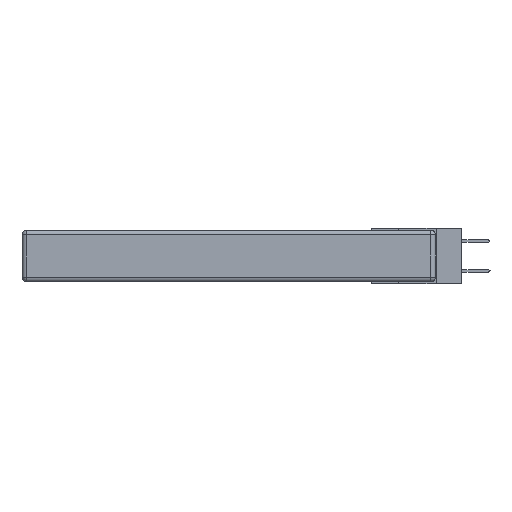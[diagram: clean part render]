
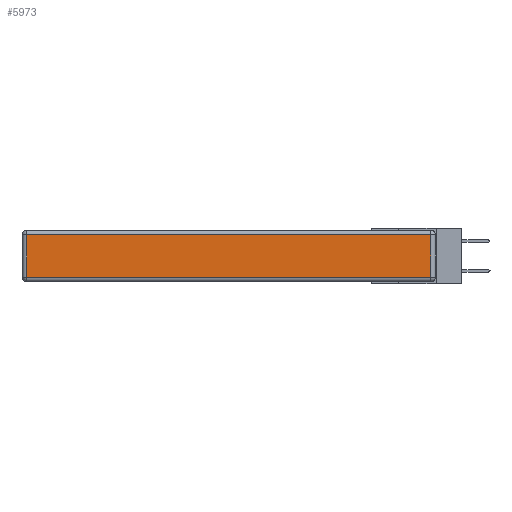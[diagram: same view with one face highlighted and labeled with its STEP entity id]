
A CAD part, left-side view. The second image highlights one B-rep face of the part: STEP entity #5973.
In plain terms, the highlighted planar face has unit normal (-1, 0, 0).
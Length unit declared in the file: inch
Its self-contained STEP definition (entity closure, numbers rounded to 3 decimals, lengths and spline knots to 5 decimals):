
#1012 = CARTESIAN_POINT ( 'NONE',  ( 0., 2.72, -0.313 ) ) ;
#1584 = VERTEX_POINT ( 'NONE', #6991 ) ;
#1770 = EDGE_CURVE ( 'NONE', #4336, #4052, #16063, .T. ) ;
#3275 = LINE ( 'NONE', #14024, #15629 ) ;
#3792 = EDGE_CURVE ( 'NONE', #1584, #4336, #3275, .T. ) ;
#3843 = DIRECTION ( 'NONE',  ( 0., 0., 1. ) ) ;
#4052 = VERTEX_POINT ( 'NONE', #1012 ) ;
#4117 = DIRECTION ( 'NONE',  ( 0., -1., 0. ) ) ;
#4202 = ORIENTED_EDGE ( 'NONE', *, *, #3792, .T. ) ;
#4336 = VERTEX_POINT ( 'NONE', #8910 ) ;
#4570 = LINE ( 'NONE', #5046, #12831 ) ;
#4706 = AXIS2_PLACEMENT_3D ( 'NONE', #4869, #13753, #10066 ) ;
#4869 = CARTESIAN_POINT ( 'NONE',  ( 0., 0., -0.343 ) ) ;
#5046 = CARTESIAN_POINT ( 'NONE',  ( 0., 0.03, -0.343 ) ) ;
#5492 = CARTESIAN_POINT ( 'NONE',  ( 0., 2.72, -0.343 ) ) ;
#5973 = ADVANCED_FACE ( 'NONE', ( #14237 ), #5983, .T. ) ;
#5983 = PLANE ( 'NONE',  #4706 ) ;
#6065 = VECTOR ( 'NONE', #6809, 39.37008 ) ;
#6703 = ORIENTED_EDGE ( 'NONE', *, *, #1770, .T. ) ;
#6809 = DIRECTION ( 'NONE',  ( 0., 0., -1. ) ) ;
#6991 = CARTESIAN_POINT ( 'NONE',  ( 0., 0.03, -0.03 ) ) ;
#7710 = VECTOR ( 'NONE', #4117, 39.37008 ) ;
#8121 = EDGE_CURVE ( 'NONE', #4052, #9071, #11029, .T. ) ;
#8174 = CARTESIAN_POINT ( 'NONE',  ( 0., 0.03, -0.313 ) ) ;
#8910 = CARTESIAN_POINT ( 'NONE',  ( 0., 2.72, -0.03 ) ) ;
#9071 = VERTEX_POINT ( 'NONE', #8174 ) ;
#10066 = DIRECTION ( 'NONE',  ( 0., 0., 1. ) ) ;
#11029 = LINE ( 'NONE', #12791, #7710 ) ;
#12519 = EDGE_LOOP ( 'NONE', ( #13437, #13417, #4202, #6703 ) ) ;
#12543 = DIRECTION ( 'NONE',  ( 0., 1., 0. ) ) ;
#12791 = CARTESIAN_POINT ( 'NONE',  ( 0., 0., -0.313 ) ) ;
#12831 = VECTOR ( 'NONE', #3843, 39.37008 ) ;
#13199 = EDGE_CURVE ( 'NONE', #9071, #1584, #4570, .T. ) ;
#13417 = ORIENTED_EDGE ( 'NONE', *, *, #13199, .T. ) ;
#13437 = ORIENTED_EDGE ( 'NONE', *, *, #8121, .T. ) ;
#13753 = DIRECTION ( 'NONE',  ( -1., 0., 0. ) ) ;
#14024 = CARTESIAN_POINT ( 'NONE',  ( 0., 2.75, -0.03 ) ) ;
#14237 = FACE_OUTER_BOUND ( 'NONE', #12519, .T. ) ;
#15629 = VECTOR ( 'NONE', #12543, 39.37008 ) ;
#16063 = LINE ( 'NONE', #5492, #6065 ) ;
